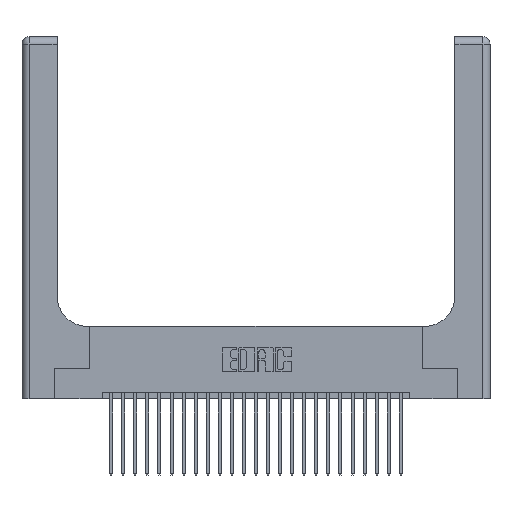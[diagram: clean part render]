
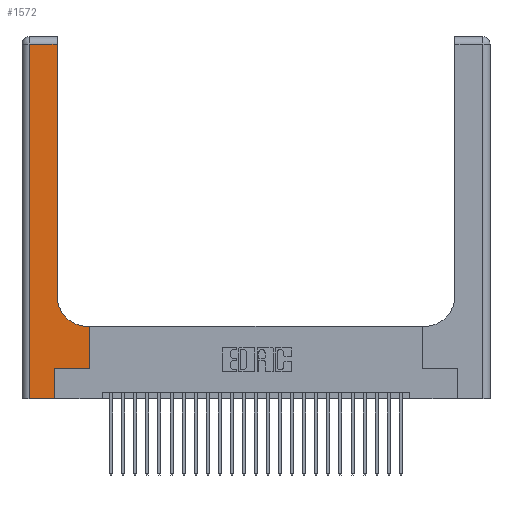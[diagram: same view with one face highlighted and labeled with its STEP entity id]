
A CAD part, top view. The second image highlights one B-rep face of the part: STEP entity #1572.
In plain terms, the highlighted planar face has unit normal (0, 0, 1).
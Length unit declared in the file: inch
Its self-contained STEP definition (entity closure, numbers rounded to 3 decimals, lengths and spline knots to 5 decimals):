
#524 = DIRECTION ( 'NONE',  ( 1., 0., 0. ) ) ;
#562 = VECTOR ( 'NONE', #14284, 39.37008 ) ;
#644 = VERTEX_POINT ( 'NONE', #20969 ) ;
#758 = EDGE_CURVE ( 'NONE', #834, #3549, #11424, .T. ) ;
#834 = VERTEX_POINT ( 'NONE', #15547 ) ;
#906 = VERTEX_POINT ( 'NONE', #15635 ) ;
#1446 = ORIENTED_EDGE ( 'NONE', *, *, #15307, .T. ) ;
#1491 = ORIENTED_EDGE ( 'NONE', *, *, #14569, .T. ) ;
#1572 = ADVANCED_FACE ( 'NONE', ( #20781 ), #5063, .F. ) ;
#1834 = CARTESIAN_POINT ( 'NONE',  ( 0.5415, 0.6, 0.37 ) ) ;
#1866 = LINE ( 'NONE', #17474, #5466 ) ;
#2169 = LINE ( 'NONE', #21406, #12265 ) ;
#2381 = VECTOR ( 'NONE', #26581, 39.37008 ) ;
#3060 = CARTESIAN_POINT ( 'NONE',  ( 0.5415, 0.85, 0.37 ) ) ;
#3189 = CARTESIAN_POINT ( 'NONE',  ( 0.2915, 3., 0.37 ) ) ;
#3549 = VERTEX_POINT ( 'NONE', #6740 ) ;
#4894 = DIRECTION ( 'NONE',  ( 1., 0., 0. ) ) ;
#5063 = PLANE ( 'NONE',  #15493 ) ;
#5149 = DIRECTION ( 'NONE',  ( 0., 0., -1. ) ) ;
#5312 = VERTEX_POINT ( 'NONE', #18388 ) ;
#5466 = VECTOR ( 'NONE', #524, 39.37008 ) ;
#5751 = VECTOR ( 'NONE', #16832, 39.37008 ) ;
#6740 = CARTESIAN_POINT ( 'NONE',  ( 0.06, 2.94, 0.37 ) ) ;
#6800 = VERTEX_POINT ( 'NONE', #1834 ) ;
#6851 = ORIENTED_EDGE ( 'NONE', *, *, #19896, .T. ) ;
#6955 = DIRECTION ( 'NONE',  ( 0., 0., -1. ) ) ;
#7387 = ORIENTED_EDGE ( 'NONE', *, *, #19197, .T. ) ;
#8590 = EDGE_CURVE ( 'NONE', #3549, #644, #12642, .T. ) ;
#8970 = DIRECTION ( 'NONE',  ( -1., 0., 0. ) ) ;
#9216 = EDGE_LOOP ( 'NONE', ( #6851, #10437, #21457, #19967, #13173, #12865, #1446, #7387, #1491 ) ) ;
#9720 = CARTESIAN_POINT ( 'NONE',  ( 0., 3., 0.37 ) ) ;
#9832 = VERTEX_POINT ( 'NONE', #16831 ) ;
#10437 = ORIENTED_EDGE ( 'NONE', *, *, #758, .T. ) ;
#11424 = LINE ( 'NONE', #12793, #21249 ) ;
#12265 = VECTOR ( 'NONE', #8970, 39.37008 ) ;
#12642 = LINE ( 'NONE', #14552, #562 ) ;
#12793 = CARTESIAN_POINT ( 'NONE',  ( 0., 2.94, 0.37 ) ) ;
#12865 = ORIENTED_EDGE ( 'NONE', *, *, #19024, .T. ) ;
#13173 = ORIENTED_EDGE ( 'NONE', *, *, #20239, .T. ) ;
#13961 = CARTESIAN_POINT ( 'NONE',  ( 0.5585, 0.25, 0.37 ) ) ;
#14048 = DIRECTION ( 'NONE',  ( 0., 1., 0. ) ) ;
#14284 = DIRECTION ( 'NONE',  ( 0., -1., 0. ) ) ;
#14552 = CARTESIAN_POINT ( 'NONE',  ( 0.06, 3., 0.37 ) ) ;
#14569 = EDGE_CURVE ( 'NONE', #6800, #9832, #22373, .T. ) ;
#14876 = LINE ( 'NONE', #26585, #25698 ) ;
#15003 = DIRECTION ( 'NONE',  ( -1., 0., 0. ) ) ;
#15307 = EDGE_CURVE ( 'NONE', #906, #20115, #17459, .T. ) ;
#15493 = AXIS2_PLACEMENT_3D ( 'NONE', #9720, #5149, #17781 ) ;
#15547 = CARTESIAN_POINT ( 'NONE',  ( 0.2915, 2.94, 0.37 ) ) ;
#15635 = CARTESIAN_POINT ( 'NONE',  ( 0.5585, 0.25, 0.37 ) ) ;
#16534 = LINE ( 'NONE', #3189, #18886 ) ;
#16831 = CARTESIAN_POINT ( 'NONE',  ( 0.2915, 0.85, 0.37 ) ) ;
#16832 = DIRECTION ( 'NONE',  ( 1., 0., 0. ) ) ;
#17459 = LINE ( 'NONE', #13961, #2381 ) ;
#17474 = CARTESIAN_POINT ( 'NONE',  ( 0., 0., 0.37 ) ) ;
#17781 = DIRECTION ( 'NONE',  ( -1., 0., 0. ) ) ;
#18388 = CARTESIAN_POINT ( 'NONE',  ( 0.269, 0., 0.37 ) ) ;
#18619 = CARTESIAN_POINT ( 'NONE',  ( 0.5585, 0.6, 0.37 ) ) ;
#18886 = VECTOR ( 'NONE', #26113, 39.37008 ) ;
#19024 = EDGE_CURVE ( 'NONE', #20478, #906, #22765, .T. ) ;
#19030 = CARTESIAN_POINT ( 'NONE',  ( 0.269, 0.25, 0.37 ) ) ;
#19197 = EDGE_CURVE ( 'NONE', #20115, #6800, #2169, .T. ) ;
#19896 = EDGE_CURVE ( 'NONE', #9832, #834, #16534, .T. ) ;
#19967 = ORIENTED_EDGE ( 'NONE', *, *, #23088, .T. ) ;
#20115 = VERTEX_POINT ( 'NONE', #18619 ) ;
#20239 = EDGE_CURVE ( 'NONE', #5312, #20478, #14876, .T. ) ;
#20478 = VERTEX_POINT ( 'NONE', #19030 ) ;
#20744 = AXIS2_PLACEMENT_3D ( 'NONE', #3060, #6955, #4894 ) ;
#20781 = FACE_OUTER_BOUND ( 'NONE', #9216, .T. ) ;
#20969 = CARTESIAN_POINT ( 'NONE',  ( 0.06, 0., 0.37 ) ) ;
#21146 = CARTESIAN_POINT ( 'NONE',  ( 0.269, 0.25, 0.37 ) ) ;
#21249 = VECTOR ( 'NONE', #15003, 39.37008 ) ;
#21406 = CARTESIAN_POINT ( 'NONE',  ( 0.2915, 0.6, 0.37 ) ) ;
#21457 = ORIENTED_EDGE ( 'NONE', *, *, #8590, .T. ) ;
#22373 = CIRCLE ( 'NONE', #20744, 0.25 ) ;
#22765 = LINE ( 'NONE', #21146, #5751 ) ;
#23088 = EDGE_CURVE ( 'NONE', #644, #5312, #1866, .T. ) ;
#25698 = VECTOR ( 'NONE', #14048, 39.37008 ) ;
#26113 = DIRECTION ( 'NONE',  ( 0., 1., 0. ) ) ;
#26581 = DIRECTION ( 'NONE',  ( 0., 1., 0. ) ) ;
#26585 = CARTESIAN_POINT ( 'NONE',  ( 0.269, 0., 0.37 ) ) ;
